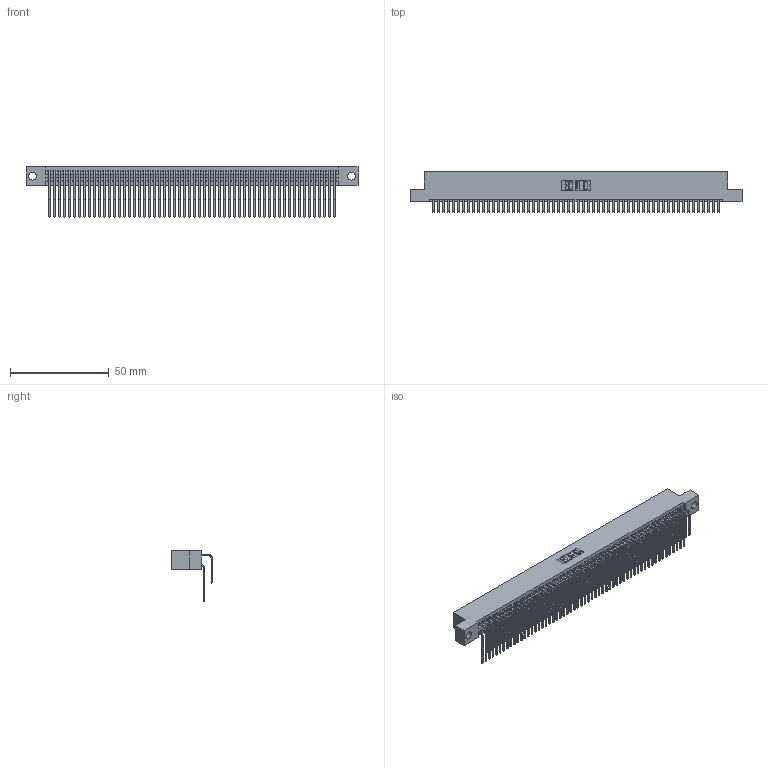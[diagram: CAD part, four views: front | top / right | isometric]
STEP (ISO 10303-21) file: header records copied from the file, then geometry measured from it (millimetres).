
FILE_DESCRIPTION (( 'STEP AP203' ), '1' );
FILE_NAME ('395-116-559-204.STEP', '2018-12-02T03:17:20', ( '' ), ( '' ), 'SwSTEP 2.0', 'SolidWorks 2016', '' );
FILE_SCHEMA (( 'CONFIG_CONTROL_DESIGN' ));
Length unit declared in the file: inch
Products named in the file (4): 345-292-001_558 559 Tail - 1; 345 Part_Flush Mounting Lugs - 0.156 Dia-TH; 345-292-001_559 Tail - 2; 395-116-559-204
Assembly tree (117 placements, depth 2):
  395-116-559-204
    345 Part_Flush Mounting Lugs - 0.156 Dia-TH
    345-292-001_558 559 Tail - 1  x58
    345-292-001_559 Tail - 2  x58
Bounding box: 168.53 x 20.56 x 25.53 mm (x, y, z)
Volume: 17100.9 mm3; surface area: 28549.8 mm2
Topology: 117 solids, 117 shells, 6158 faces, 18321 edges, 12058 vertices
Faces by surface type: plane 4140, cylinder 2018
Entity records: 45009 total; most frequent: CARTESIAN_POINT 7575, ORIENTED_EDGE 7458, DIRECTION 6633, EDGE_CURVE 3729, LINE 3325, VECTOR 3325, VERTEX_POINT 2482, AXIS2_PLACEMENT_3D 1654
